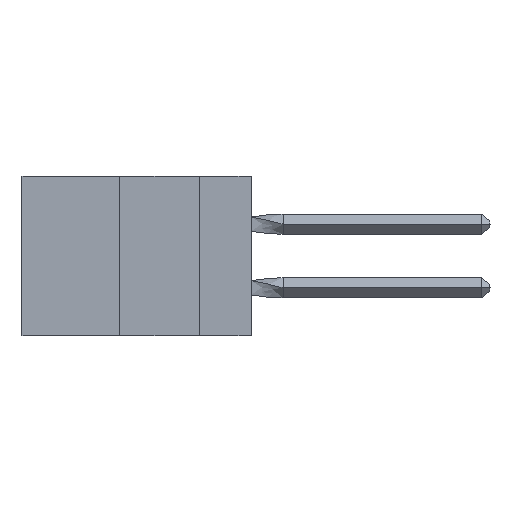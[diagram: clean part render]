
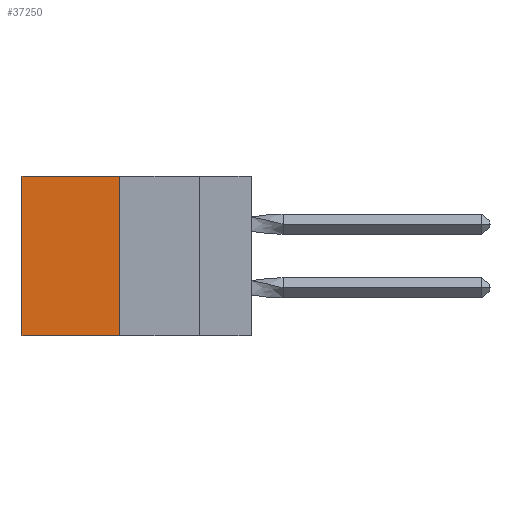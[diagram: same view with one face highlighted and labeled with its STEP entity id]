
A CAD part, left-side view. The second image highlights one B-rep face of the part: STEP entity #37250.
In plain terms, the highlighted planar face has unit normal (-1, 0, 0).
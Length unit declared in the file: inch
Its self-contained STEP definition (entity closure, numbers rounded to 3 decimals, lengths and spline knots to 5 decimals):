
#143 = AXIS2_PLACEMENT_3D ( 'NONE', #24701, #18850, #3889 ) ;
#638 = VECTOR ( 'NONE', #14077, 39.37008 ) ;
#3065 = EDGE_CURVE ( 'NONE', #12373, #35701, #31775, .T. ) ;
#3765 = PLANE ( 'NONE',  #143 ) ;
#3889 = DIRECTION ( 'NONE',  ( 0., 0., -1. ) ) ;
#5425 = VECTOR ( 'NONE', #25394, 39.37008 ) ;
#6253 = LINE ( 'NONE', #18501, #26310 ) ;
#6930 = EDGE_CURVE ( 'NONE', #26869, #34865, #32681, .T. ) ;
#8942 = FACE_OUTER_BOUND ( 'NONE', #30560, .T. ) ;
#11343 = CARTESIAN_POINT ( 'NONE',  ( 0.305, 0.72, 0. ) ) ;
#12373 = VERTEX_POINT ( 'NONE', #21512 ) ;
#12527 = ORIENTED_EDGE ( 'NONE', *, *, #3065, .T. ) ;
#13472 = ORIENTED_EDGE ( 'NONE', *, *, #26031, .F. ) ;
#14077 = DIRECTION ( 'NONE',  ( 0., 0., -1. ) ) ;
#14434 = CARTESIAN_POINT ( 'NONE',  ( 0.305, 0.413, 0. ) ) ;
#16152 = ORIENTED_EDGE ( 'NONE', *, *, #6930, .F. ) ;
#16353 = CARTESIAN_POINT ( 'NONE',  ( 0.305, 0.72, -0.5 ) ) ;
#18501 = CARTESIAN_POINT ( 'NONE',  ( 0.305, 0.72, -0.5 ) ) ;
#18850 = DIRECTION ( 'NONE',  ( 1., 0., 0. ) ) ;
#20469 = EDGE_CURVE ( 'NONE', #35701, #34865, #6253, .T. ) ;
#20550 = CARTESIAN_POINT ( 'NONE',  ( 0.305, 0.413, -0.5 ) ) ;
#21170 = LINE ( 'NONE', #22716, #638 ) ;
#21512 = CARTESIAN_POINT ( 'NONE',  ( 0.305, 0.413, 0. ) ) ;
#22716 = CARTESIAN_POINT ( 'NONE',  ( 0.305, 0.413, -0.5 ) ) ;
#23356 = DIRECTION ( 'NONE',  ( 0., 1., 0. ) ) ;
#24701 = CARTESIAN_POINT ( 'NONE',  ( 0.305, 0.413, -0.5 ) ) ;
#25394 = DIRECTION ( 'NONE',  ( 0., 1., 0. ) ) ;
#26031 = EDGE_CURVE ( 'NONE', #12373, #26869, #21170, .T. ) ;
#26310 = VECTOR ( 'NONE', #28096, 39.37008 ) ;
#26869 = VERTEX_POINT ( 'NONE', #20550 ) ;
#28096 = DIRECTION ( 'NONE',  ( 0., 0., -1. ) ) ;
#30560 = EDGE_LOOP ( 'NONE', ( #33143, #16152, #13472, #12527 ) ) ;
#31775 = LINE ( 'NONE', #14434, #37067 ) ;
#32681 = LINE ( 'NONE', #37338, #5425 ) ;
#33143 = ORIENTED_EDGE ( 'NONE', *, *, #20469, .T. ) ;
#34865 = VERTEX_POINT ( 'NONE', #16353 ) ;
#35701 = VERTEX_POINT ( 'NONE', #11343 ) ;
#37067 = VECTOR ( 'NONE', #23356, 39.37008 ) ;
#37250 = ADVANCED_FACE ( 'NONE', ( #8942 ), #3765, .F. ) ;
#37338 = CARTESIAN_POINT ( 'NONE',  ( 0.305, 0.413, -0.5 ) ) ;
